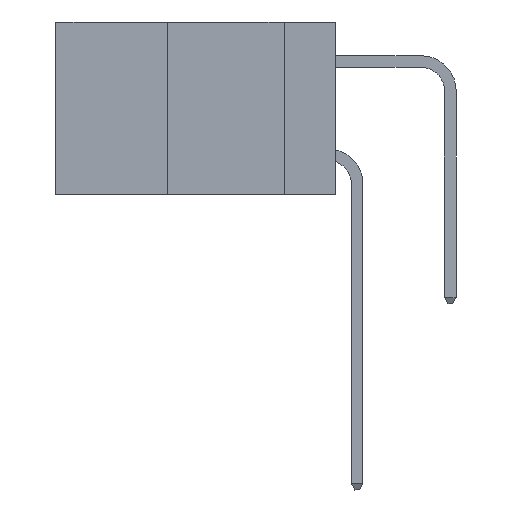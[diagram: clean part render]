
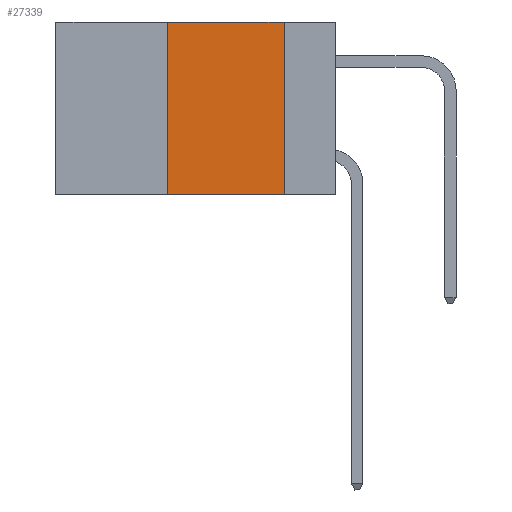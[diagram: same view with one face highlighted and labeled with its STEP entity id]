
A CAD part, left-side view. The second image highlights one B-rep face of the part: STEP entity #27339.
In plain terms, the highlighted planar face has unit normal (-1, 0, 0).
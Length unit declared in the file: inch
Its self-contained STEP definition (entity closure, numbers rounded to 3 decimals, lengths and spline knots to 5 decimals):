
#1498 = VERTEX_POINT ( 'NONE', #27567 ) ;
#1554 = VECTOR ( 'NONE', #24199, 39.37008 ) ;
#2854 = CARTESIAN_POINT ( 'NONE',  ( 0., 0.6, 0. ) ) ;
#5302 = PLANE ( 'NONE',  #22783 ) ;
#5353 = VERTEX_POINT ( 'NONE', #33949 ) ;
#6199 = DIRECTION ( 'NONE',  ( 0., -1., 0. ) ) ;
#7860 = CARTESIAN_POINT ( 'NONE',  ( 0., 0.6, -0.37 ) ) ;
#9787 = EDGE_LOOP ( 'NONE', ( #39636, #29214, #40137, #21097 ) ) ;
#10164 = DIRECTION ( 'NONE',  ( 0., 0., 1. ) ) ;
#10431 = LINE ( 'NONE', #7860, #1554 ) ;
#11996 = CARTESIAN_POINT ( 'NONE',  ( 0., 0.6, 0. ) ) ;
#13163 = EDGE_CURVE ( 'NONE', #1498, #5353, #10431, .T. ) ;
#13912 = LINE ( 'NONE', #2854, #30033 ) ;
#15258 = DIRECTION ( 'NONE',  ( 0., 0., -1. ) ) ;
#16296 = DIRECTION ( 'NONE',  ( 0., 0., -1. ) ) ;
#18185 = LINE ( 'NONE', #29538, #34251 ) ;
#19197 = FACE_OUTER_BOUND ( 'NONE', #9787, .T. ) ;
#21097 = ORIENTED_EDGE ( 'NONE', *, *, #13163, .T. ) ;
#22783 = AXIS2_PLACEMENT_3D ( 'NONE', #11996, #34495, #15258 ) ;
#22815 = VECTOR ( 'NONE', #16296, 39.37008 ) ;
#24199 = DIRECTION ( 'NONE',  ( 0., -1., 0. ) ) ;
#24510 = CARTESIAN_POINT ( 'NONE',  ( 0., 0.36, 0. ) ) ;
#24647 = CARTESIAN_POINT ( 'NONE',  ( 0., 0.11, 0. ) ) ;
#26133 = EDGE_CURVE ( 'NONE', #36126, #5353, #40815, .T. ) ;
#26920 = EDGE_CURVE ( 'NONE', #1498, #33395, #18185, .T. ) ;
#27339 = ADVANCED_FACE ( 'NONE', ( #19197 ), #5302, .F. ) ;
#27567 = CARTESIAN_POINT ( 'NONE',  ( 0., 0.36, -0.37 ) ) ;
#29214 = ORIENTED_EDGE ( 'NONE', *, *, #30356, .F. ) ;
#29538 = CARTESIAN_POINT ( 'NONE',  ( 0., 0.36, 0. ) ) ;
#30033 = VECTOR ( 'NONE', #6199, 39.37008 ) ;
#30356 = EDGE_CURVE ( 'NONE', #33395, #36126, #13912, .T. ) ;
#32322 = CARTESIAN_POINT ( 'NONE',  ( 0., 0.11, 0. ) ) ;
#33395 = VERTEX_POINT ( 'NONE', #24510 ) ;
#33949 = CARTESIAN_POINT ( 'NONE',  ( 0., 0.11, -0.37 ) ) ;
#34251 = VECTOR ( 'NONE', #10164, 39.37008 ) ;
#34495 = DIRECTION ( 'NONE',  ( 1., 0., 0. ) ) ;
#36126 = VERTEX_POINT ( 'NONE', #24647 ) ;
#39636 = ORIENTED_EDGE ( 'NONE', *, *, #26133, .F. ) ;
#40137 = ORIENTED_EDGE ( 'NONE', *, *, #26920, .F. ) ;
#40815 = LINE ( 'NONE', #32322, #22815 ) ;
